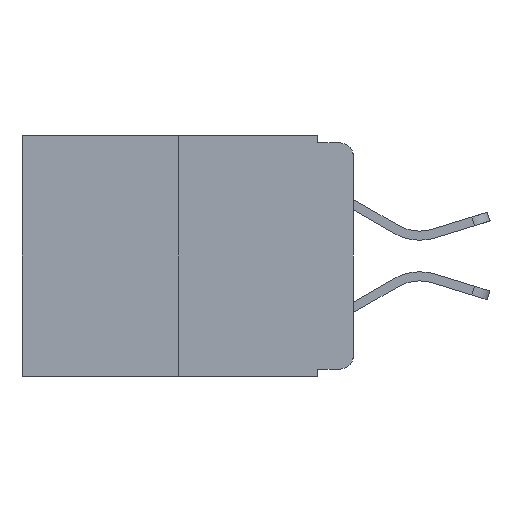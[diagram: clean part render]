
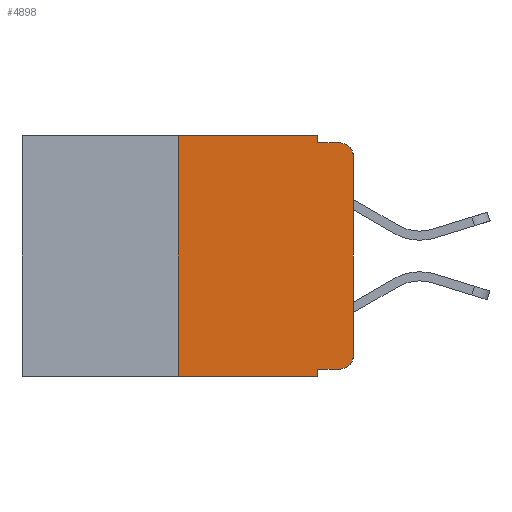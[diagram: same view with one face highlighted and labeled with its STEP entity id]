
A CAD part, left-side view. The second image highlights one B-rep face of the part: STEP entity #4898.
In plain terms, the highlighted planar face has unit normal (-1, 0, 0).
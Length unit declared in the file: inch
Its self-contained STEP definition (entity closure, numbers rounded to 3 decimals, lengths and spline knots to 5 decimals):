
#61 = CARTESIAN_POINT ( 'NONE',  ( 0., 0.02, -0.01 ) ) ;
#94 = EDGE_CURVE ( 'NONE', #3553, #8062, #9357, .T. ) ;
#153 = VECTOR ( 'NONE', #3226, 39.37008 ) ;
#320 = DIRECTION ( 'NONE',  ( 0., 0., 1. ) ) ;
#458 = DIRECTION ( 'NONE',  ( 0., -1., 0. ) ) ;
#486 = ORIENTED_EDGE ( 'NONE', *, *, #8362, .F. ) ;
#499 = PLANE ( 'NONE',  #8804 ) ;
#572 = VERTEX_POINT ( 'NONE', #61 ) ;
#641 = DIRECTION ( 'NONE',  ( 0., 0., -1. ) ) ;
#815 = CARTESIAN_POINT ( 'NONE',  ( 0., 0.02, -0.333 ) ) ;
#1008 = VECTOR ( 'NONE', #320, 39.37008 ) ;
#1129 = LINE ( 'NONE', #9433, #7285 ) ;
#1160 = CIRCLE ( 'NONE', #3386, 0.02 ) ;
#1267 = LINE ( 'NONE', #1276, #9789 ) ;
#1276 = CARTESIAN_POINT ( 'NONE',  ( 0., 0.051, -0.01 ) ) ;
#1310 = ORIENTED_EDGE ( 'NONE', *, *, #94, .T. ) ;
#1487 = VECTOR ( 'NONE', #9685, 39.37008 ) ;
#1746 = LINE ( 'NONE', #4859, #1487 ) ;
#1806 = VECTOR ( 'NONE', #5509, 39.37008 ) ;
#1809 = VERTEX_POINT ( 'NONE', #5060 ) ;
#1980 = ORIENTED_EDGE ( 'NONE', *, *, #8515, .T. ) ;
#2236 = CARTESIAN_POINT ( 'NONE',  ( 0., 0.051, 0. ) ) ;
#2255 = DIRECTION ( 'NONE',  ( 1., 0., 0. ) ) ;
#2258 = ORIENTED_EDGE ( 'NONE', *, *, #8440, .F. ) ;
#2329 = CARTESIAN_POINT ( 'NONE',  ( 0., 0.25, -0.343 ) ) ;
#2757 = VECTOR ( 'NONE', #3093, 39.37008 ) ;
#2779 = FACE_OUTER_BOUND ( 'NONE', #4437, .T. ) ;
#2795 = EDGE_CURVE ( 'NONE', #8500, #1809, #1746, .T. ) ;
#2833 = VECTOR ( 'NONE', #458, 39.37008 ) ;
#2931 = DIRECTION ( 'NONE',  ( 0., 0., -1. ) ) ;
#3093 = DIRECTION ( 'NONE',  ( 0., 0., -1. ) ) ;
#3226 = DIRECTION ( 'NONE',  ( 0., 0., 1. ) ) ;
#3303 = LINE ( 'NONE', #8647, #1008 ) ;
#3326 = ORIENTED_EDGE ( 'NONE', *, *, #7853, .F. ) ;
#3386 = AXIS2_PLACEMENT_3D ( 'NONE', #9227, #4367, #10032 ) ;
#3553 = VERTEX_POINT ( 'NONE', #5530 ) ;
#3653 = CARTESIAN_POINT ( 'NONE',  ( 0., 0.25, 0. ) ) ;
#3949 = CARTESIAN_POINT ( 'NONE',  ( 0., 0.051, -0.01 ) ) ;
#4367 = DIRECTION ( 'NONE',  ( -1., 0., 0. ) ) ;
#4437 = EDGE_LOOP ( 'NONE', ( #1980, #8578, #2258, #8824, #486, #5306, #9581, #3326, #1310, #5814 ) ) ;
#4574 = EDGE_CURVE ( 'NONE', #10689, #572, #1160, .T. ) ;
#4672 = CARTESIAN_POINT ( 'NONE',  ( 0., 0.473, 0. ) ) ;
#4836 = CARTESIAN_POINT ( 'NONE',  ( 0., 0., -0.03 ) ) ;
#4859 = CARTESIAN_POINT ( 'NONE',  ( 0., 0.473, -0.343 ) ) ;
#4898 = ADVANCED_FACE ( 'NONE', ( #2779 ), #499, .F. ) ;
#4969 = EDGE_CURVE ( 'NONE', #8062, #7775, #8061, .T. ) ;
#5060 = CARTESIAN_POINT ( 'NONE',  ( 0., 0.051, -0.343 ) ) ;
#5306 = ORIENTED_EDGE ( 'NONE', *, *, #5885, .F. ) ;
#5509 = DIRECTION ( 'NONE',  ( 0., -1., 0. ) ) ;
#5530 = CARTESIAN_POINT ( 'NONE',  ( 0., 0.051, -0.333 ) ) ;
#5615 = DIRECTION ( 'NONE',  ( 0., -1., 0. ) ) ;
#5742 = DIRECTION ( 'NONE',  ( -1., 0., 0. ) ) ;
#5814 = ORIENTED_EDGE ( 'NONE', *, *, #4969, .T. ) ;
#5815 = VERTEX_POINT ( 'NONE', #3653 ) ;
#5885 = EDGE_CURVE ( 'NONE', #8500, #5815, #3303, .T. ) ;
#6288 = LINE ( 'NONE', #4672, #1806 ) ;
#6575 = EDGE_CURVE ( 'NONE', #9271, #6708, #1129, .T. ) ;
#6708 = VERTEX_POINT ( 'NONE', #3949 ) ;
#6920 = LINE ( 'NONE', #7340, #153 ) ;
#7285 = VECTOR ( 'NONE', #2931, 39.37008 ) ;
#7340 = CARTESIAN_POINT ( 'NONE',  ( 0., 0., 0. ) ) ;
#7734 = CARTESIAN_POINT ( 'NONE',  ( 0., 0.051, -0.333 ) ) ;
#7775 = VERTEX_POINT ( 'NONE', #8718 ) ;
#7853 = EDGE_CURVE ( 'NONE', #3553, #1809, #9282, .T. ) ;
#7885 = CARTESIAN_POINT ( 'NONE',  ( 0., 0.051, 0. ) ) ;
#8041 = DIRECTION ( 'NONE',  ( 0., 0., -1. ) ) ;
#8061 = CIRCLE ( 'NONE', #9344, 0.02 ) ;
#8062 = VERTEX_POINT ( 'NONE', #815 ) ;
#8362 = EDGE_CURVE ( 'NONE', #5815, #9271, #6288, .T. ) ;
#8440 = EDGE_CURVE ( 'NONE', #6708, #572, #1267, .T. ) ;
#8500 = VERTEX_POINT ( 'NONE', #2329 ) ;
#8515 = EDGE_CURVE ( 'NONE', #7775, #10689, #6920, .T. ) ;
#8578 = ORIENTED_EDGE ( 'NONE', *, *, #4574, .T. ) ;
#8647 = CARTESIAN_POINT ( 'NONE',  ( 0., 0.25, 0. ) ) ;
#8718 = CARTESIAN_POINT ( 'NONE',  ( 0., 0., -0.313 ) ) ;
#8804 = AXIS2_PLACEMENT_3D ( 'NONE', #9614, #2255, #8041 ) ;
#8824 = ORIENTED_EDGE ( 'NONE', *, *, #6575, .F. ) ;
#9227 = CARTESIAN_POINT ( 'NONE',  ( 0., 0.02, -0.03 ) ) ;
#9271 = VERTEX_POINT ( 'NONE', #7885 ) ;
#9282 = LINE ( 'NONE', #2236, #2757 ) ;
#9344 = AXIS2_PLACEMENT_3D ( 'NONE', #10567, #5742, #641 ) ;
#9357 = LINE ( 'NONE', #7734, #2833 ) ;
#9433 = CARTESIAN_POINT ( 'NONE',  ( 0., 0.051, 0. ) ) ;
#9581 = ORIENTED_EDGE ( 'NONE', *, *, #2795, .T. ) ;
#9614 = CARTESIAN_POINT ( 'NONE',  ( 0., 0.473, 0. ) ) ;
#9685 = DIRECTION ( 'NONE',  ( 0., -1., 0. ) ) ;
#9789 = VECTOR ( 'NONE', #5615, 39.37008 ) ;
#10032 = DIRECTION ( 'NONE',  ( 0., 0., -1. ) ) ;
#10567 = CARTESIAN_POINT ( 'NONE',  ( 0., 0.02, -0.313 ) ) ;
#10689 = VERTEX_POINT ( 'NONE', #4836 ) ;
